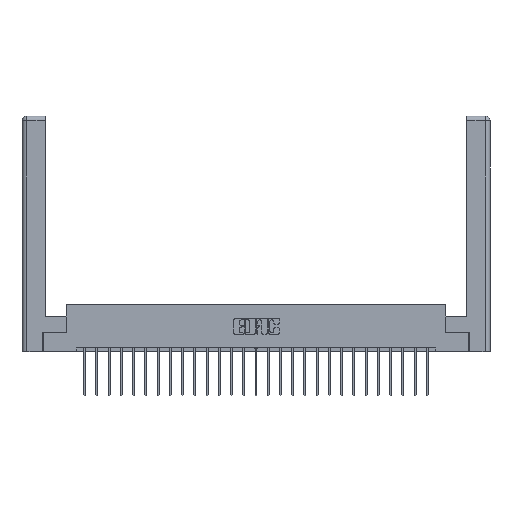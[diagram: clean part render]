
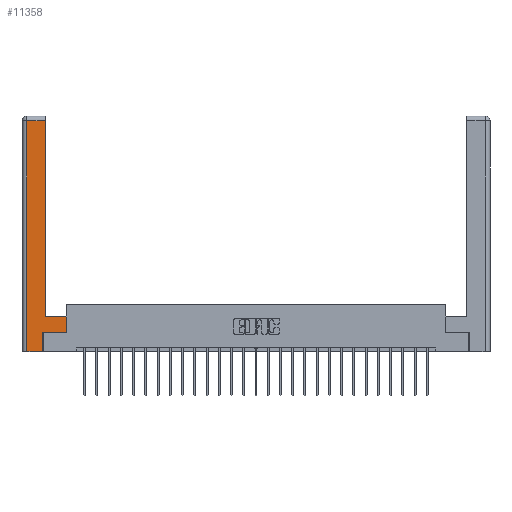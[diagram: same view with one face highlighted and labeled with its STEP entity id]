
A CAD part, top view. The second image highlights one B-rep face of the part: STEP entity #11358.
In plain terms, the highlighted planar face has unit normal (0, 0, 1).
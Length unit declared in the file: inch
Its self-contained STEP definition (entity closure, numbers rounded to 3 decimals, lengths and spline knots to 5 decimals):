
#63 = LINE ( 'NONE', #15286, #26641 ) ;
#557 = DIRECTION ( 'NONE',  ( -1., 0., 0. ) ) ;
#585 = CARTESIAN_POINT ( 'NONE',  ( 0.565, 0.245, 0. ) ) ;
#952 = DIRECTION ( 'NONE',  ( 1., 0., 0. ) ) ;
#1800 = EDGE_CURVE ( 'NONE', #22161, #4744, #22932, .T. ) ;
#2960 = ORIENTED_EDGE ( 'NONE', *, *, #10567, .T. ) ;
#3496 = EDGE_LOOP ( 'NONE', ( #15115, #9523, #8241, #25549, #23893, #2960, #13403, #3943 ) ) ;
#3843 = CARTESIAN_POINT ( 'NONE',  ( 0.565, 0.245, 0. ) ) ;
#3943 = ORIENTED_EDGE ( 'NONE', *, *, #23758, .T. ) ;
#4351 = CARTESIAN_POINT ( 'NONE',  ( 0.265, 0.245, 0. ) ) ;
#4383 = LINE ( 'NONE', #24149, #25830 ) ;
#4744 = VERTEX_POINT ( 'NONE', #11082 ) ;
#4810 = CARTESIAN_POINT ( 'NONE',  ( 0.0615, 0., 0. ) ) ;
#5336 = EDGE_CURVE ( 'NONE', #8798, #21426, #63, .T. ) ;
#5514 = DIRECTION ( 'NONE',  ( 0., 1., 0. ) ) ;
#6098 = AXIS2_PLACEMENT_3D ( 'NONE', #19225, #21325, #10979 ) ;
#6101 = LINE ( 'NONE', #8295, #11619 ) ;
#6128 = LINE ( 'NONE', #22917, #15868 ) ;
#6624 = EDGE_CURVE ( 'NONE', #17716, #8798, #9096, .T. ) ;
#7647 = CARTESIAN_POINT ( 'NONE',  ( 0.295, 0.45, 0. ) ) ;
#8241 = ORIENTED_EDGE ( 'NONE', *, *, #23594, .T. ) ;
#8295 = CARTESIAN_POINT ( 'NONE',  ( 0.295, 0.45, 0. ) ) ;
#8303 = CARTESIAN_POINT ( 'NONE',  ( 0.565, 0.45, 0. ) ) ;
#8727 = PLANE ( 'NONE',  #6098 ) ;
#8798 = VERTEX_POINT ( 'NONE', #25555 ) ;
#9096 = LINE ( 'NONE', #21089, #16523 ) ;
#9523 = ORIENTED_EDGE ( 'NONE', *, *, #17659, .T. ) ;
#10567 = EDGE_CURVE ( 'NONE', #21426, #22161, #12737, .T. ) ;
#10979 = DIRECTION ( 'NONE',  ( -1., 0., 0. ) ) ;
#11082 = CARTESIAN_POINT ( 'NONE',  ( 0.565, 0.45, 0. ) ) ;
#11358 = ADVANCED_FACE ( 'NONE', ( #23419 ), #8727, .F. ) ;
#11567 = VECTOR ( 'NONE', #12420, 39.37008 ) ;
#11619 = VECTOR ( 'NONE', #16729, 39.37008 ) ;
#12123 = DIRECTION ( 'NONE',  ( 0., -1., 0. ) ) ;
#12420 = DIRECTION ( 'NONE',  ( 0., 1., 0. ) ) ;
#12737 = LINE ( 'NONE', #585, #15035 ) ;
#13403 = ORIENTED_EDGE ( 'NONE', *, *, #1800, .T. ) ;
#14553 = CARTESIAN_POINT ( 'NONE',  ( 0.295, 2.94, 0. ) ) ;
#15035 = VECTOR ( 'NONE', #952, 39.37008 ) ;
#15115 = ORIENTED_EDGE ( 'NONE', *, *, #19192, .T. ) ;
#15144 = LINE ( 'NONE', #24894, #11567 ) ;
#15286 = CARTESIAN_POINT ( 'NONE',  ( 0.265, 0.245, 0. ) ) ;
#15868 = VECTOR ( 'NONE', #12123, 39.37008 ) ;
#16523 = VECTOR ( 'NONE', #17009, 39.37008 ) ;
#16729 = DIRECTION ( 'NONE',  ( -1., 0., 0. ) ) ;
#17009 = DIRECTION ( 'NONE',  ( 1., 0., 0. ) ) ;
#17407 = VECTOR ( 'NONE', #5514, 39.37008 ) ;
#17487 = VERTEX_POINT ( 'NONE', #14553 ) ;
#17643 = CARTESIAN_POINT ( 'NONE',  ( 0.0615, 2.94, 0. ) ) ;
#17659 = EDGE_CURVE ( 'NONE', #17487, #25768, #4383, .T. ) ;
#17716 = VERTEX_POINT ( 'NONE', #4810 ) ;
#19192 = EDGE_CURVE ( 'NONE', #21189, #17487, #15144, .T. ) ;
#19225 = CARTESIAN_POINT ( 'NONE',  ( 0., 0., 0. ) ) ;
#19816 = DIRECTION ( 'NONE',  ( 0., 1., 0. ) ) ;
#21089 = CARTESIAN_POINT ( 'NONE',  ( 0.265, 0., 0. ) ) ;
#21189 = VERTEX_POINT ( 'NONE', #7647 ) ;
#21325 = DIRECTION ( 'NONE',  ( 0., 0., -1. ) ) ;
#21426 = VERTEX_POINT ( 'NONE', #4351 ) ;
#22161 = VERTEX_POINT ( 'NONE', #3843 ) ;
#22917 = CARTESIAN_POINT ( 'NONE',  ( 0.0615, 0., 0. ) ) ;
#22932 = LINE ( 'NONE', #8303, #17407 ) ;
#23419 = FACE_OUTER_BOUND ( 'NONE', #3496, .T. ) ;
#23594 = EDGE_CURVE ( 'NONE', #25768, #17716, #6128, .T. ) ;
#23758 = EDGE_CURVE ( 'NONE', #4744, #21189, #6101, .T. ) ;
#23893 = ORIENTED_EDGE ( 'NONE', *, *, #5336, .T. ) ;
#24149 = CARTESIAN_POINT ( 'NONE',  ( 0.0615, 2.94, 0. ) ) ;
#24894 = CARTESIAN_POINT ( 'NONE',  ( 0.295, 3., 0. ) ) ;
#25549 = ORIENTED_EDGE ( 'NONE', *, *, #6624, .T. ) ;
#25555 = CARTESIAN_POINT ( 'NONE',  ( 0.265, 0., 0. ) ) ;
#25768 = VERTEX_POINT ( 'NONE', #17643 ) ;
#25830 = VECTOR ( 'NONE', #557, 39.37008 ) ;
#26641 = VECTOR ( 'NONE', #19816, 39.37008 ) ;
